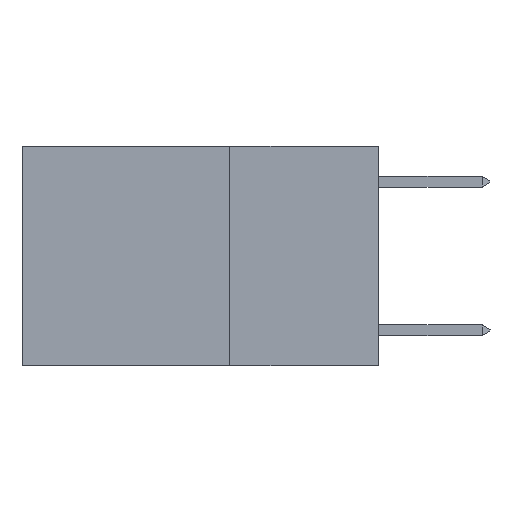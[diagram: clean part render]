
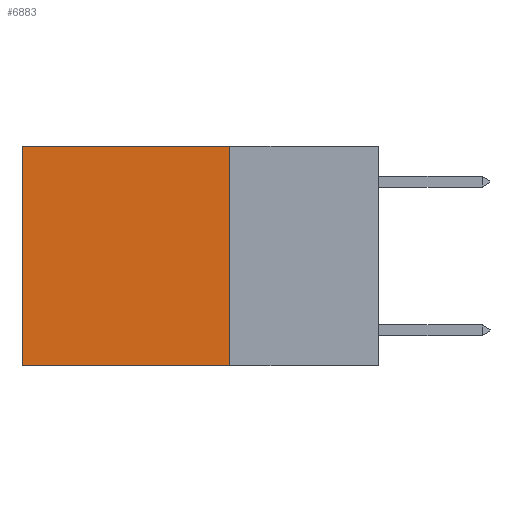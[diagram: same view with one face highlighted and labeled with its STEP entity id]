
A CAD part, left-side view. The second image highlights one B-rep face of the part: STEP entity #6883.
In plain terms, the highlighted planar face has unit normal (-1, 0, 0).
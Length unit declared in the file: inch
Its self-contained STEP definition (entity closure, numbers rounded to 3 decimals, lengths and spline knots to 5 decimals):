
#1071 = LINE ( 'NONE', #4179, #11176 ) ;
#1561 = LINE ( 'NONE', #28557, #25987 ) ;
#2427 = VERTEX_POINT ( 'NONE', #21167 ) ;
#2433 = EDGE_CURVE ( 'NONE', #2427, #14647, #4133, .T. ) ;
#4133 = LINE ( 'NONE', #4302, #24196 ) ;
#4179 = CARTESIAN_POINT ( 'NONE',  ( 0.2625, 0.25, -0.37 ) ) ;
#4242 = VERTEX_POINT ( 'NONE', #9312 ) ;
#4302 = CARTESIAN_POINT ( 'NONE',  ( 0.2625, 0.25, 0. ) ) ;
#4563 = VERTEX_POINT ( 'NONE', #30668 ) ;
#4816 = AXIS2_PLACEMENT_3D ( 'NONE', #17695, #15297, #27024 ) ;
#4942 = ORIENTED_EDGE ( 'NONE', *, *, #10272, .F. ) ;
#6735 = DIRECTION ( 'NONE',  ( 0., 1., 0. ) ) ;
#6883 = ADVANCED_FACE ( 'NONE', ( #19641 ), #27346, .F. ) ;
#7736 = ORIENTED_EDGE ( 'NONE', *, *, #28080, .T. ) ;
#9054 = CARTESIAN_POINT ( 'NONE',  ( 0.2625, 0.6, 0. ) ) ;
#9312 = CARTESIAN_POINT ( 'NONE',  ( 0.2625, 0.6, 0. ) ) ;
#10272 = EDGE_CURVE ( 'NONE', #14647, #4563, #1071, .T. ) ;
#10715 = DIRECTION ( 'NONE',  ( 0., 1., 0. ) ) ;
#10980 = VECTOR ( 'NONE', #14541, 39.37008 ) ;
#11176 = VECTOR ( 'NONE', #6735, 39.37008 ) ;
#13942 = DIRECTION ( 'NONE',  ( 0., 0., -1. ) ) ;
#14541 = DIRECTION ( 'NONE',  ( 0., 0., -1. ) ) ;
#14647 = VERTEX_POINT ( 'NONE', #23574 ) ;
#15297 = DIRECTION ( 'NONE',  ( 1., 0., 0. ) ) ;
#17695 = CARTESIAN_POINT ( 'NONE',  ( 0.2625, 0.25, 0. ) ) ;
#18849 = EDGE_CURVE ( 'NONE', #4242, #4563, #26577, .T. ) ;
#19641 = FACE_OUTER_BOUND ( 'NONE', #28672, .T. ) ;
#21167 = CARTESIAN_POINT ( 'NONE',  ( 0.2625, 0.25, 0. ) ) ;
#23574 = CARTESIAN_POINT ( 'NONE',  ( 0.2625, 0.25, -0.37 ) ) ;
#24059 = ORIENTED_EDGE ( 'NONE', *, *, #2433, .F. ) ;
#24196 = VECTOR ( 'NONE', #13942, 39.37008 ) ;
#25987 = VECTOR ( 'NONE', #10715, 39.37008 ) ;
#26577 = LINE ( 'NONE', #9054, #10980 ) ;
#27024 = DIRECTION ( 'NONE',  ( 0., 0., -1. ) ) ;
#27346 = PLANE ( 'NONE',  #4816 ) ;
#28080 = EDGE_CURVE ( 'NONE', #2427, #4242, #1561, .T. ) ;
#28557 = CARTESIAN_POINT ( 'NONE',  ( 0.2625, 0.25, 0. ) ) ;
#28672 = EDGE_LOOP ( 'NONE', ( #30508, #4942, #24059, #7736 ) ) ;
#30508 = ORIENTED_EDGE ( 'NONE', *, *, #18849, .T. ) ;
#30668 = CARTESIAN_POINT ( 'NONE',  ( 0.2625, 0.6, -0.37 ) ) ;
